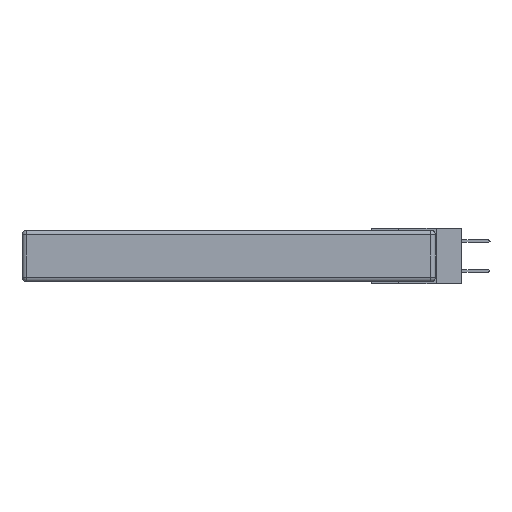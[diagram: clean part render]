
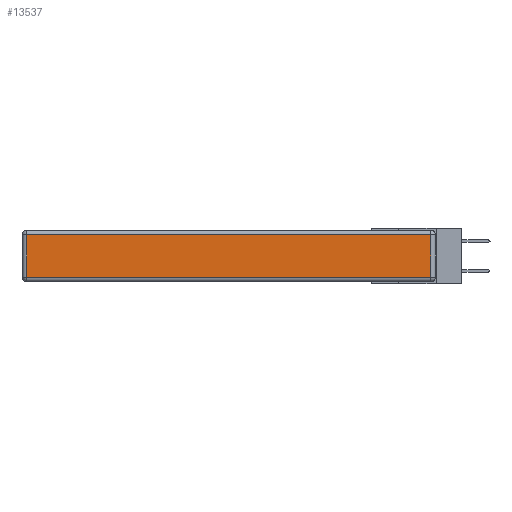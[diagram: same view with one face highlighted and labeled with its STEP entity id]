
A CAD part, left-side view. The second image highlights one B-rep face of the part: STEP entity #13537.
In plain terms, the highlighted planar face has unit normal (-1, 0, 0).
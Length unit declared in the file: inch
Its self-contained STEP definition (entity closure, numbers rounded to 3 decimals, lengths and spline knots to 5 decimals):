
#659 = EDGE_CURVE ( 'NONE', #17958, #17190, #27487, .T. ) ;
#2096 = CARTESIAN_POINT ( 'NONE',  ( 0., 2.75, -0.03 ) ) ;
#2454 = CARTESIAN_POINT ( 'NONE',  ( 0., 2.72, -0.03 ) ) ;
#2777 = VECTOR ( 'NONE', #21240, 39.37008 ) ;
#4321 = VECTOR ( 'NONE', #17507, 39.37008 ) ;
#5222 = VERTEX_POINT ( 'NONE', #28836 ) ;
#6167 = ORIENTED_EDGE ( 'NONE', *, *, #12284, .T. ) ;
#7288 = DIRECTION ( 'NONE',  ( 0., -1., 0. ) ) ;
#8348 = ORIENTED_EDGE ( 'NONE', *, *, #27117, .T. ) ;
#8435 = DIRECTION ( 'NONE',  ( -1., 0., 0. ) ) ;
#8658 = CARTESIAN_POINT ( 'NONE',  ( 0., 0.03, -0.313 ) ) ;
#10504 = DIRECTION ( 'NONE',  ( 0., 1., 0. ) ) ;
#11540 = DIRECTION ( 'NONE',  ( 0., 0., 1. ) ) ;
#12109 = CARTESIAN_POINT ( 'NONE',  ( 0., 2.72, -0.343 ) ) ;
#12284 = EDGE_CURVE ( 'NONE', #5222, #29342, #25060, .T. ) ;
#12882 = EDGE_CURVE ( 'NONE', #17190, #5222, #18512, .T. ) ;
#13537 = ADVANCED_FACE ( 'NONE', ( #31377 ), #16955, .T. ) ;
#14964 = EDGE_LOOP ( 'NONE', ( #6167, #8348, #23737, #29474 ) ) ;
#15545 = CARTESIAN_POINT ( 'NONE',  ( 0., 0.03, -0.343 ) ) ;
#16356 = VECTOR ( 'NONE', #7288, 39.37008 ) ;
#16955 = PLANE ( 'NONE',  #17898 ) ;
#17190 = VERTEX_POINT ( 'NONE', #2454 ) ;
#17507 = DIRECTION ( 'NONE',  ( 0., 0., -1. ) ) ;
#17898 = AXIS2_PLACEMENT_3D ( 'NONE', #27882, #8435, #11540 ) ;
#17958 = VERTEX_POINT ( 'NONE', #26133 ) ;
#18512 = LINE ( 'NONE', #12109, #4321 ) ;
#21240 = DIRECTION ( 'NONE',  ( 0., 0., 1. ) ) ;
#23433 = LINE ( 'NONE', #15545, #2777 ) ;
#23737 = ORIENTED_EDGE ( 'NONE', *, *, #659, .T. ) ;
#25060 = LINE ( 'NONE', #30820, #16356 ) ;
#26133 = CARTESIAN_POINT ( 'NONE',  ( 0., 0.03, -0.03 ) ) ;
#27117 = EDGE_CURVE ( 'NONE', #29342, #17958, #23433, .T. ) ;
#27487 = LINE ( 'NONE', #2096, #30044 ) ;
#27882 = CARTESIAN_POINT ( 'NONE',  ( 0., 0., -0.343 ) ) ;
#28836 = CARTESIAN_POINT ( 'NONE',  ( 0., 2.72, -0.313 ) ) ;
#29342 = VERTEX_POINT ( 'NONE', #8658 ) ;
#29474 = ORIENTED_EDGE ( 'NONE', *, *, #12882, .T. ) ;
#30044 = VECTOR ( 'NONE', #10504, 39.37008 ) ;
#30820 = CARTESIAN_POINT ( 'NONE',  ( 0., 0., -0.313 ) ) ;
#31377 = FACE_OUTER_BOUND ( 'NONE', #14964, .T. ) ;
